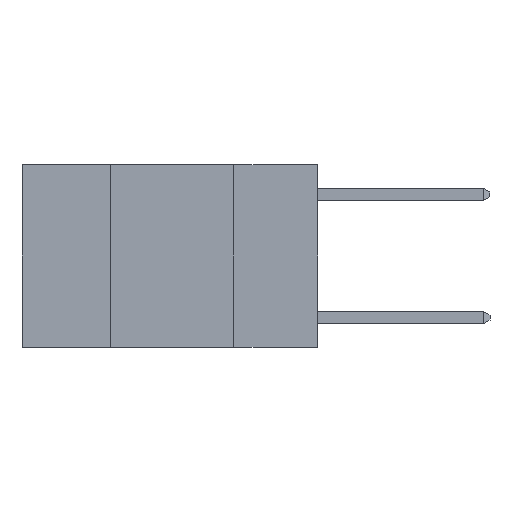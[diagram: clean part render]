
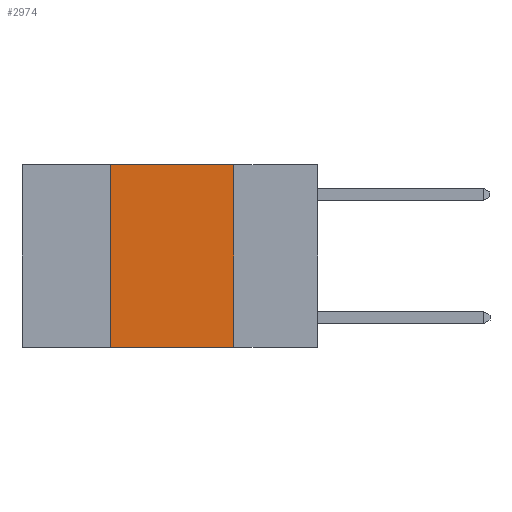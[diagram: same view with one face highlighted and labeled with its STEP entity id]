
A CAD part, left-side view. The second image highlights one B-rep face of the part: STEP entity #2974.
In plain terms, the highlighted planar face has unit normal (-1, 0, 0).
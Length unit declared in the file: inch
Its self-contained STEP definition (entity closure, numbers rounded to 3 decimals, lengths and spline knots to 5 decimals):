
#105 = EDGE_LOOP ( 'NONE', ( #8205, #6120, #584, #2041 ) ) ;
#168 = LINE ( 'NONE', #3115, #5269 ) ;
#584 = ORIENTED_EDGE ( 'NONE', *, *, #1946, .F. ) ;
#1132 = CARTESIAN_POINT ( 'NONE',  ( 0., 0.6, 0. ) ) ;
#1420 = DIRECTION ( 'NONE',  ( 0., -1., 0. ) ) ;
#1582 = DIRECTION ( 'NONE',  ( 0., 0., -1. ) ) ;
#1685 = VECTOR ( 'NONE', #1420, 39.37008 ) ;
#1820 = DIRECTION ( 'NONE',  ( 0., 0., -1. ) ) ;
#1857 = CARTESIAN_POINT ( 'NONE',  ( 0., 0.17, -0.37 ) ) ;
#1946 = EDGE_CURVE ( 'NONE', #2508, #3555, #168, .T. ) ;
#2019 = LINE ( 'NONE', #5706, #6688 ) ;
#2041 = ORIENTED_EDGE ( 'NONE', *, *, #6025, .T. ) ;
#2508 = VERTEX_POINT ( 'NONE', #8657 ) ;
#2542 = DIRECTION ( 'NONE',  ( 1., 0., 0. ) ) ;
#2782 = PLANE ( 'NONE',  #7857 ) ;
#2974 = ADVANCED_FACE ( 'NONE', ( #8485 ), #2782, .F. ) ;
#3115 = CARTESIAN_POINT ( 'NONE',  ( 0., 0.42, 0. ) ) ;
#3144 = CARTESIAN_POINT ( 'NONE',  ( 0., 0.42, 0. ) ) ;
#3272 = LINE ( 'NONE', #6050, #1685 ) ;
#3555 = VERTEX_POINT ( 'NONE', #3144 ) ;
#3586 = VECTOR ( 'NONE', #1582, 39.37008 ) ;
#4253 = VERTEX_POINT ( 'NONE', #1857 ) ;
#5269 = VECTOR ( 'NONE', #6550, 39.37008 ) ;
#5598 = VERTEX_POINT ( 'NONE', #6172 ) ;
#5706 = CARTESIAN_POINT ( 'NONE',  ( 0., 0.6, 0. ) ) ;
#5802 = EDGE_CURVE ( 'NONE', #3555, #5598, #2019, .T. ) ;
#6025 = EDGE_CURVE ( 'NONE', #2508, #4253, #3272, .T. ) ;
#6050 = CARTESIAN_POINT ( 'NONE',  ( 0., 0.6, -0.37 ) ) ;
#6120 = ORIENTED_EDGE ( 'NONE', *, *, #5802, .F. ) ;
#6172 = CARTESIAN_POINT ( 'NONE',  ( 0., 0.17, 0. ) ) ;
#6209 = EDGE_CURVE ( 'NONE', #5598, #4253, #7308, .T. ) ;
#6219 = CARTESIAN_POINT ( 'NONE',  ( 0., 0.17, 0. ) ) ;
#6318 = DIRECTION ( 'NONE',  ( 0., -1., 0. ) ) ;
#6550 = DIRECTION ( 'NONE',  ( 0., 0., 1. ) ) ;
#6688 = VECTOR ( 'NONE', #6318, 39.37008 ) ;
#7308 = LINE ( 'NONE', #6219, #3586 ) ;
#7857 = AXIS2_PLACEMENT_3D ( 'NONE', #1132, #2542, #1820 ) ;
#8205 = ORIENTED_EDGE ( 'NONE', *, *, #6209, .F. ) ;
#8485 = FACE_OUTER_BOUND ( 'NONE', #105, .T. ) ;
#8657 = CARTESIAN_POINT ( 'NONE',  ( 0., 0.42, -0.37 ) ) ;
